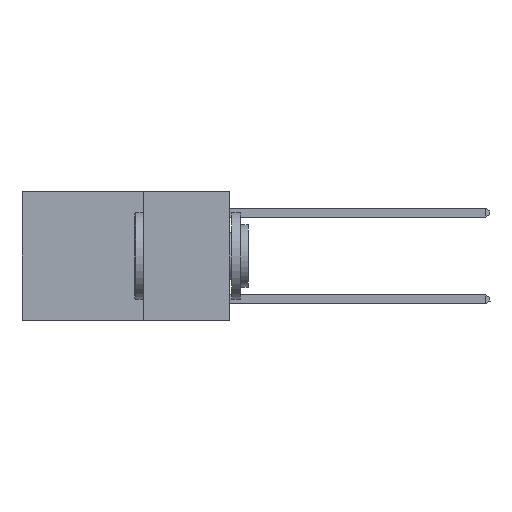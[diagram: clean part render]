
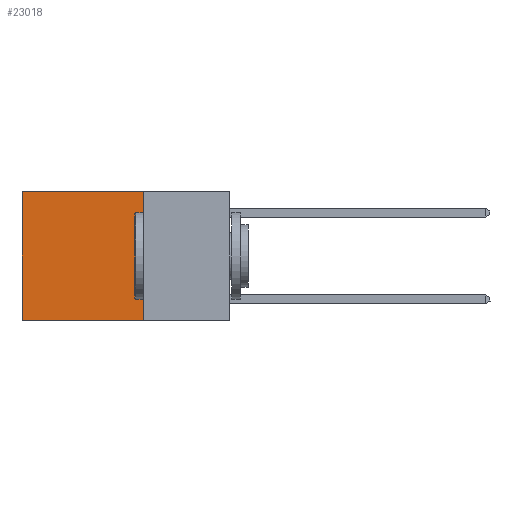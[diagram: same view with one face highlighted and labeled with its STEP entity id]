
A CAD part, left-side view. The second image highlights one B-rep face of the part: STEP entity #23018.
In plain terms, the highlighted planar face has unit normal (-1, 0, 0).
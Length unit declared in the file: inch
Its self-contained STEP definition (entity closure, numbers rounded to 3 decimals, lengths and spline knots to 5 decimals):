
#1111 = CARTESIAN_POINT ( 'NONE',  ( 0.2625, 0.25, 0. ) ) ;
#1582 = CARTESIAN_POINT ( 'NONE',  ( 0.2625, 0.6, 0. ) ) ;
#2281 = EDGE_CURVE ( 'NONE', #14322, #20499, #19813, .T. ) ;
#2436 = VERTEX_POINT ( 'NONE', #1582 ) ;
#2551 = LINE ( 'NONE', #10034, #26621 ) ;
#2713 = FACE_OUTER_BOUND ( 'NONE', #9566, .T. ) ;
#2731 = DIRECTION ( 'NONE',  ( 0., 0., -1. ) ) ;
#2883 = DIRECTION ( 'NONE',  ( 0., 1., 0. ) ) ;
#3016 = VECTOR ( 'NONE', #14315, 39.37008 ) ;
#3649 = CARTESIAN_POINT ( 'NONE',  ( 0.2625, 0.25, -0.37 ) ) ;
#5778 = ORIENTED_EDGE ( 'NONE', *, *, #14245, .T. ) ;
#8533 = LINE ( 'NONE', #1111, #22410 ) ;
#9566 = EDGE_LOOP ( 'NONE', ( #5778, #27677, #29467, #27905 ) ) ;
#10034 = CARTESIAN_POINT ( 'NONE',  ( 0.2625, 0.25, -0.37 ) ) ;
#10686 = DIRECTION ( 'NONE',  ( 0., 0., -1. ) ) ;
#14245 = EDGE_CURVE ( 'NONE', #2436, #23285, #17283, .T. ) ;
#14315 = DIRECTION ( 'NONE',  ( 0., 0., -1. ) ) ;
#14322 = VERTEX_POINT ( 'NONE', #27084 ) ;
#15316 = CARTESIAN_POINT ( 'NONE',  ( 0.2625, 0.25, 0. ) ) ;
#15461 = CARTESIAN_POINT ( 'NONE',  ( 0.2625, 0.25, 0. ) ) ;
#17283 = LINE ( 'NONE', #27245, #3016 ) ;
#18470 = DIRECTION ( 'NONE',  ( 0., 1., 0. ) ) ;
#19813 = LINE ( 'NONE', #15316, #32594 ) ;
#20499 = VERTEX_POINT ( 'NONE', #3649 ) ;
#22396 = CARTESIAN_POINT ( 'NONE',  ( 0.2625, 0.6, -0.37 ) ) ;
#22410 = VECTOR ( 'NONE', #18470, 39.37008 ) ;
#23018 = ADVANCED_FACE ( 'NONE', ( #2713 ), #30711, .F. ) ;
#23285 = VERTEX_POINT ( 'NONE', #22396 ) ;
#24041 = EDGE_CURVE ( 'NONE', #20499, #23285, #2551, .T. ) ;
#25951 = DIRECTION ( 'NONE',  ( 1., 0., 0. ) ) ;
#26621 = VECTOR ( 'NONE', #2883, 39.37008 ) ;
#27084 = CARTESIAN_POINT ( 'NONE',  ( 0.2625, 0.25, 0. ) ) ;
#27245 = CARTESIAN_POINT ( 'NONE',  ( 0.2625, 0.6, 0. ) ) ;
#27677 = ORIENTED_EDGE ( 'NONE', *, *, #24041, .F. ) ;
#27760 = AXIS2_PLACEMENT_3D ( 'NONE', #15461, #25951, #10686 ) ;
#27905 = ORIENTED_EDGE ( 'NONE', *, *, #28478, .T. ) ;
#28478 = EDGE_CURVE ( 'NONE', #14322, #2436, #8533, .T. ) ;
#29467 = ORIENTED_EDGE ( 'NONE', *, *, #2281, .F. ) ;
#30711 = PLANE ( 'NONE',  #27760 ) ;
#32594 = VECTOR ( 'NONE', #2731, 39.37008 ) ;
